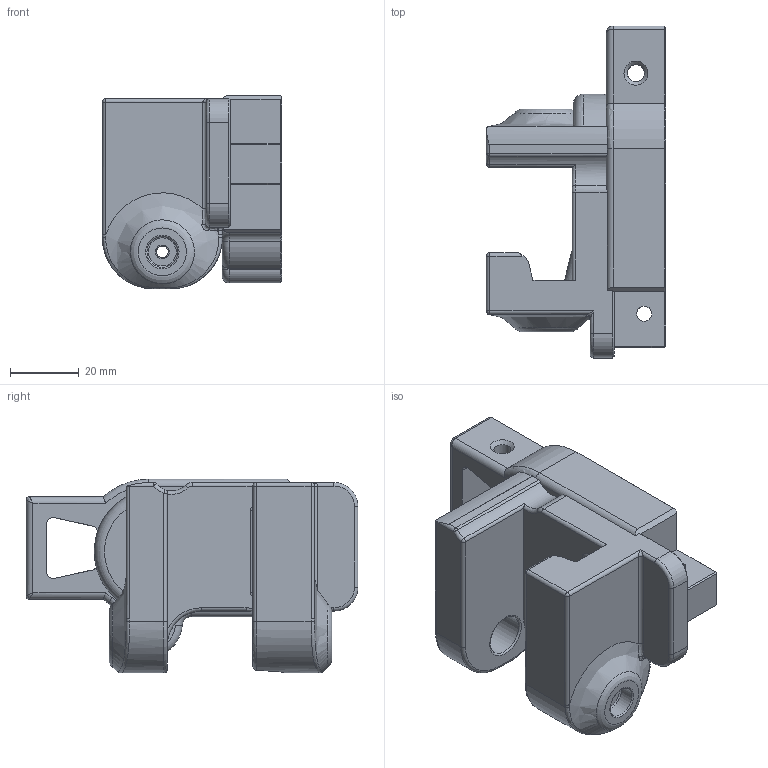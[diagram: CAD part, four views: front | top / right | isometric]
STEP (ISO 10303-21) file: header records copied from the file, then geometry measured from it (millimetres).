
FILE_DESCRIPTION (( 'STEP AP203' ), '1' );
FILE_NAME ('MOD9_endcap.STEP', '2020-06-10T04:58:43', ( '' ), ( '' ), 'SwSTEP 2.0', 'SolidWorks 2016', '' );
FILE_SCHEMA (( 'CONFIG_CONTROL_DESIGN' ));
Length unit declared in the file: millimetre
Products named in the file (1): MOD9_endcap
Bounding box: 52.33 x 96.9 x 56.54 mm (x, y, z)
Volume: 108439.3 mm3; surface area: 25719.8 mm2
Topology: 1 solids, 1 shells, 231 faces, 577 edges, 347 vertices
Faces by surface type: plane 81, cylinder 71, torus 31, bspline 22, cone 21, sphere 5
Full cylindrical faces by diameter (mm): 3.4 x1, 4 x1, 4.4 x1, 5 x2, 9 x1, 12 x1, 23 x1
Entity records: 7934 total; most frequent: CARTESIAN_POINT 2727, ORIENTED_EDGE 1092, DIRECTION 997, EDGE_CURVE 546, AXIS2_PLACEMENT_3D 372, VERTEX_POINT 341, EDGE_LOOP 267, LINE 253
